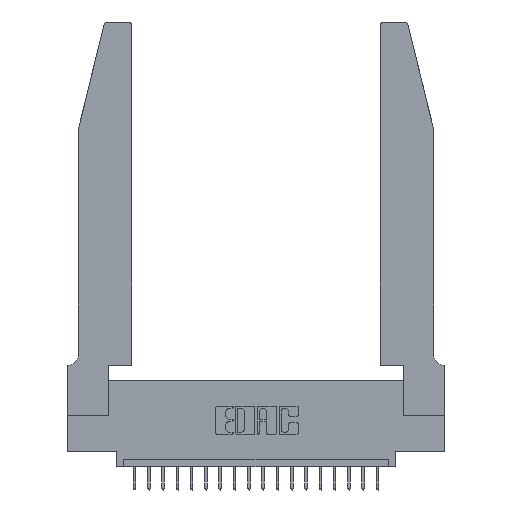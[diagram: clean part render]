
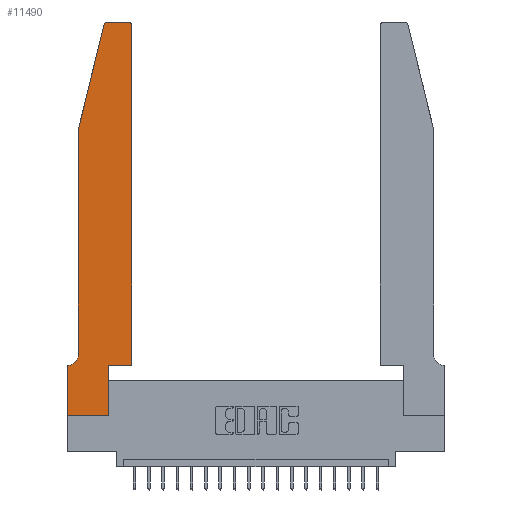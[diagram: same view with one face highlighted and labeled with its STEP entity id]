
A CAD part, top view. The second image highlights one B-rep face of the part: STEP entity #11490.
In plain terms, the highlighted planar face has unit normal (0, 0, 1).
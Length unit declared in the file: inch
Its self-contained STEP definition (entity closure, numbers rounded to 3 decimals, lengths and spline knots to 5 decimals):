
#4 = VERTEX_POINT ( 'NONE', #14313 ) ;
#144 = DIRECTION ( 'NONE',  ( 1., 0., 0. ) ) ;
#365 = EDGE_CURVE ( 'NONE', #14505, #4, #12662, .T. ) ;
#436 = CARTESIAN_POINT ( 'NONE',  ( 0.4505, 2.72, 0.37 ) ) ;
#598 = ORIENTED_EDGE ( 'NONE', *, *, #11109, .T. ) ;
#709 = AXIS2_PLACEMENT_3D ( 'NONE', #19025, #20698, #16107 ) ;
#870 = LINE ( 'NONE', #16381, #18190 ) ;
#933 = VECTOR ( 'NONE', #2238, 39.37008 ) ;
#1021 = VERTEX_POINT ( 'NONE', #7359 ) ;
#1169 = CARTESIAN_POINT ( 'NONE',  ( 0.2865, 0.35, 0.37 ) ) ;
#1321 = VECTOR ( 'NONE', #9890, 39.37008 ) ;
#1378 = CARTESIAN_POINT ( 'NONE',  ( 0., 0.35, 0.37 ) ) ;
#1662 = CARTESIAN_POINT ( 'NONE',  ( 0.2865, 0., 0.37 ) ) ;
#1833 = VECTOR ( 'NONE', #15488, 39.37008 ) ;
#1902 = EDGE_CURVE ( 'NONE', #13361, #1021, #6548, .T. ) ;
#2067 = VECTOR ( 'NONE', #12952, 39.37008 ) ;
#2238 = DIRECTION ( 'NONE',  ( -0.239, -0.971, 0. ) ) ;
#2367 = EDGE_CURVE ( 'NONE', #1021, #17819, #16242, .T. ) ;
#2434 = VECTOR ( 'NONE', #19658, 39.37008 ) ;
#2839 = VERTEX_POINT ( 'NONE', #13790 ) ;
#3242 = EDGE_CURVE ( 'NONE', #2839, #15132, #12054, .T. ) ;
#3454 = CARTESIAN_POINT ( 'NONE',  ( 0.4505, 0.35, 0.37 ) ) ;
#3466 = CARTESIAN_POINT ( 'NONE',  ( 0.0055, 0.35, 0.37 ) ) ;
#3788 = CARTESIAN_POINT ( 'NONE',  ( 0., 0., 0.37 ) ) ;
#4100 = LINE ( 'NONE', #12343, #933 ) ;
#4711 = CARTESIAN_POINT ( 'NONE',  ( 0.2865, 0.35, 0.37 ) ) ;
#4888 = VERTEX_POINT ( 'NONE', #1169 ) ;
#5015 = CARTESIAN_POINT ( 'NONE',  ( 0.284, 2.72, 0.37 ) ) ;
#5895 = ORIENTED_EDGE ( 'NONE', *, *, #18687, .T. ) ;
#6074 = ORIENTED_EDGE ( 'NONE', *, *, #19429, .T. ) ;
#6107 = VERTEX_POINT ( 'NONE', #436 ) ;
#6245 = EDGE_CURVE ( 'NONE', #7408, #14505, #870, .T. ) ;
#6495 = ORIENTED_EDGE ( 'NONE', *, *, #13002, .T. ) ;
#6520 = CARTESIAN_POINT ( 'NONE',  ( 0., 0., 0.37 ) ) ;
#6548 = LINE ( 'NONE', #7805, #2067 ) ;
#6641 = FACE_OUTER_BOUND ( 'NONE', #19785, .T. ) ;
#7359 = CARTESIAN_POINT ( 'NONE',  ( 0.284, 2.75, 0.37 ) ) ;
#7408 = VERTEX_POINT ( 'NONE', #3466 ) ;
#7460 = DIRECTION ( 'NONE',  ( 0., 1., 0. ) ) ;
#7535 = DIRECTION ( 'NONE',  ( 0., 0., -1. ) ) ;
#7777 = AXIS2_PLACEMENT_3D ( 'NONE', #5015, #11881, #8365 ) ;
#7805 = CARTESIAN_POINT ( 'NONE',  ( 0.2605, 2.75, 0.37 ) ) ;
#7853 = CIRCLE ( 'NONE', #709, 0.03 ) ;
#7869 = CIRCLE ( 'NONE', #13614, 0.07 ) ;
#7982 = LINE ( 'NONE', #4711, #2434 ) ;
#8161 = ORIENTED_EDGE ( 'NONE', *, *, #365, .T. ) ;
#8365 = DIRECTION ( 'NONE',  ( 1., 0., 0. ) ) ;
#8750 = EDGE_CURVE ( 'NONE', #15132, #7408, #7869, .T. ) ;
#9119 = DIRECTION ( 'NONE',  ( -1., 0., 0. ) ) ;
#9343 = EDGE_CURVE ( 'NONE', #19066, #6107, #16739, .T. ) ;
#9464 = CARTESIAN_POINT ( 'NONE',  ( 0.25487, 2.72718, 0.37 ) ) ;
#9890 = DIRECTION ( 'NONE',  ( 1., 0., 0. ) ) ;
#10717 = CARTESIAN_POINT ( 'NONE',  ( 0.4505, 0.35, 0.37 ) ) ;
#11056 = DIRECTION ( 'NONE',  ( 0., -1., 0. ) ) ;
#11109 = EDGE_CURVE ( 'NONE', #4888, #19066, #14315, .T. ) ;
#11415 = ORIENTED_EDGE ( 'NONE', *, *, #3242, .T. ) ;
#11490 = ADVANCED_FACE ( 'NONE', ( #6641 ), #14762, .T. ) ;
#11622 = DIRECTION ( 'NONE',  ( 1., 0., 0. ) ) ;
#11683 = CARTESIAN_POINT ( 'NONE',  ( 0.4505, 0.35, 0.37 ) ) ;
#11797 = CARTESIAN_POINT ( 'NONE',  ( 0.0755, 2., 0.37 ) ) ;
#11881 = DIRECTION ( 'NONE',  ( 0., 0., 1. ) ) ;
#12054 = LINE ( 'NONE', #11797, #20354 ) ;
#12343 = CARTESIAN_POINT ( 'NONE',  ( 0.0755, 2., 0.37 ) ) ;
#12662 = LINE ( 'NONE', #3788, #1833 ) ;
#12737 = CARTESIAN_POINT ( 'NONE',  ( 0.4205, 2.75, 0.37 ) ) ;
#12952 = DIRECTION ( 'NONE',  ( -1., 0., 0. ) ) ;
#13002 = EDGE_CURVE ( 'NONE', #4, #13922, #17866, .T. ) ;
#13112 = DIRECTION ( 'NONE',  ( -1., 0., 0. ) ) ;
#13162 = DIRECTION ( 'NONE',  ( 0., 0., 1. ) ) ;
#13361 = VERTEX_POINT ( 'NONE', #12737 ) ;
#13614 = AXIS2_PLACEMENT_3D ( 'NONE', #19093, #7535, #9119 ) ;
#13790 = CARTESIAN_POINT ( 'NONE',  ( 0.0755, 2., 0.37 ) ) ;
#13922 = VERTEX_POINT ( 'NONE', #1662 ) ;
#14027 = VECTOR ( 'NONE', #144, 39.37008 ) ;
#14313 = CARTESIAN_POINT ( 'NONE',  ( 0., 0., 0.37 ) ) ;
#14315 = LINE ( 'NONE', #3454, #14027 ) ;
#14377 = CARTESIAN_POINT ( 'NONE',  ( 0., 0.35, 0.37 ) ) ;
#14505 = VERTEX_POINT ( 'NONE', #14377 ) ;
#14762 = PLANE ( 'NONE',  #16859 ) ;
#15119 = ORIENTED_EDGE ( 'NONE', *, *, #1902, .T. ) ;
#15132 = VERTEX_POINT ( 'NONE', #18518 ) ;
#15464 = VECTOR ( 'NONE', #7460, 39.37008 ) ;
#15488 = DIRECTION ( 'NONE',  ( 0., -1., 0. ) ) ;
#16107 = DIRECTION ( 'NONE',  ( 1., 0., 0. ) ) ;
#16242 = CIRCLE ( 'NONE', #7777, 0.03 ) ;
#16381 = CARTESIAN_POINT ( 'NONE',  ( 0.0755, 0.35, 0.37 ) ) ;
#16621 = ORIENTED_EDGE ( 'NONE', *, *, #17199, .T. ) ;
#16739 = LINE ( 'NONE', #10717, #15464 ) ;
#16859 = AXIS2_PLACEMENT_3D ( 'NONE', #1378, #13162, #11622 ) ;
#17199 = EDGE_CURVE ( 'NONE', #13922, #4888, #7982, .T. ) ;
#17819 = VERTEX_POINT ( 'NONE', #9464 ) ;
#17866 = LINE ( 'NONE', #6520, #1321 ) ;
#18190 = VECTOR ( 'NONE', #13112, 39.37008 ) ;
#18518 = CARTESIAN_POINT ( 'NONE',  ( 0.0755, 0.42, 0.37 ) ) ;
#18687 = EDGE_CURVE ( 'NONE', #6107, #13361, #7853, .T. ) ;
#19025 = CARTESIAN_POINT ( 'NONE',  ( 0.4205, 2.72, 0.37 ) ) ;
#19066 = VERTEX_POINT ( 'NONE', #11683 ) ;
#19093 = CARTESIAN_POINT ( 'NONE',  ( 0.0055, 0.42, 0.37 ) ) ;
#19429 = EDGE_CURVE ( 'NONE', #17819, #2839, #4100, .T. ) ;
#19658 = DIRECTION ( 'NONE',  ( 0., 1., 0. ) ) ;
#19702 = ORIENTED_EDGE ( 'NONE', *, *, #2367, .T. ) ;
#19785 = EDGE_LOOP ( 'NONE', ( #15119, #19702, #6074, #11415, #20333, #20879, #8161, #6495, #16621, #598, #21243, #5895 ) ) ;
#20333 = ORIENTED_EDGE ( 'NONE', *, *, #8750, .T. ) ;
#20354 = VECTOR ( 'NONE', #11056, 39.37008 ) ;
#20698 = DIRECTION ( 'NONE',  ( 0., 0., 1. ) ) ;
#20879 = ORIENTED_EDGE ( 'NONE', *, *, #6245, .T. ) ;
#21243 = ORIENTED_EDGE ( 'NONE', *, *, #9343, .T. ) ;
